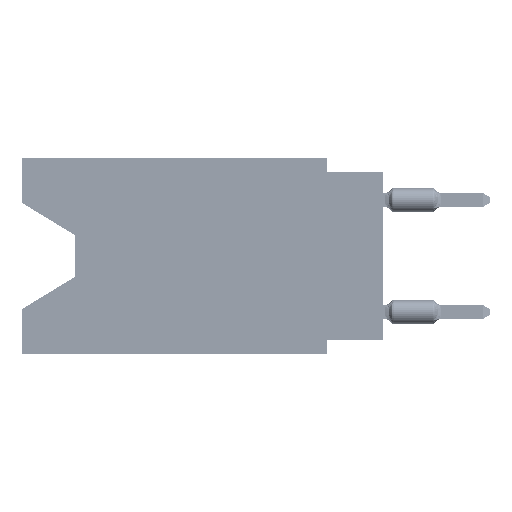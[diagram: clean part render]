
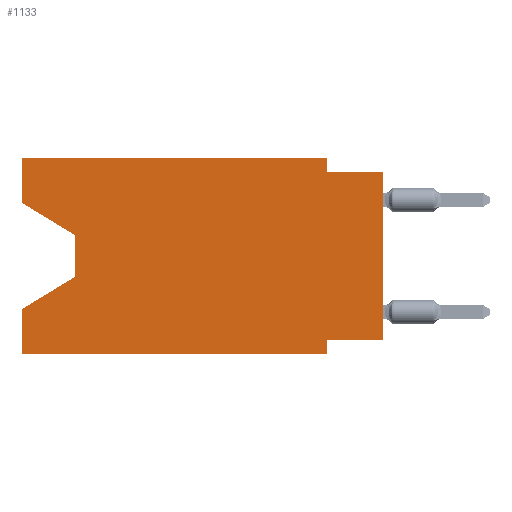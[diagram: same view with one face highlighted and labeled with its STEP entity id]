
A CAD part, left-side view. The second image highlights one B-rep face of the part: STEP entity #1133.
In plain terms, the highlighted planar face has unit normal (-1, 0, 0).
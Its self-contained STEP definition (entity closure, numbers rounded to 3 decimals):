
#1133 = ADVANCED_FACE ( 'NONE', ( #46735 ), #67381, .F. ) ;
#1563 = CARTESIAN_POINT ( 'NONE',  ( 0., 16.383, 0. ) ) ;
#1635 = CARTESIAN_POINT ( 'NONE',  ( 0., 0., -0.635 ) ) ;
#2254 = VERTEX_POINT ( 'NONE', #71745 ) ;
#2310 = VERTEX_POINT ( 'NONE', #57102 ) ;
#2483 = CARTESIAN_POINT ( 'NONE',  ( 0., 13.97, -5.385 ) ) ;
#3102 = VERTEX_POINT ( 'NONE', #33386 ) ;
#5741 = EDGE_LOOP ( 'NONE', ( #50713, #13413, #11217, #46353, #14247, #51278, #54764, #56738, #67167, #51960, #11838, #71206 ) ) ;
#6582 = EDGE_CURVE ( 'NONE', #58281, #15753, #70233, .T. ) ;
#9421 = VECTOR ( 'NONE', #40419, 1000. ) ;
#9939 = CARTESIAN_POINT ( 'NONE',  ( 0., 16.383, -6.852 ) ) ;
#10693 = LINE ( 'NONE', #43326, #68741 ) ;
#11217 = ORIENTED_EDGE ( 'NONE', *, *, #6582, .T. ) ;
#11391 = DIRECTION ( 'NONE',  ( 0., 0., -1. ) ) ;
#11838 = ORIENTED_EDGE ( 'NONE', *, *, #20810, .F. ) ;
#13413 = ORIENTED_EDGE ( 'NONE', *, *, #21229, .T. ) ;
#13521 = DIRECTION ( 'NONE',  ( 0., 0., 1. ) ) ;
#13876 = LINE ( 'NONE', #63709, #57979 ) ;
#14247 = ORIENTED_EDGE ( 'NONE', *, *, #32171, .T. ) ;
#14319 = CARTESIAN_POINT ( 'NONE',  ( 0., 16.383, -8.89 ) ) ;
#14470 = DIRECTION ( 'NONE',  ( 0., 0., -1. ) ) ;
#15527 = VECTOR ( 'NONE', #39495, 1000. ) ;
#15753 = VERTEX_POINT ( 'NONE', #9939 ) ;
#16280 = LINE ( 'NONE', #55493, #27519 ) ;
#16481 = VECTOR ( 'NONE', #11391, 1000. ) ;
#16884 = CARTESIAN_POINT ( 'NONE',  ( 0., 13.97, -3.505 ) ) ;
#20309 = CARTESIAN_POINT ( 'NONE',  ( 0., 13.97, -5.385 ) ) ;
#20413 = LINE ( 'NONE', #42416, #56230 ) ;
#20764 = EDGE_CURVE ( 'NONE', #67572, #26858, #44441, .T. ) ;
#20810 = EDGE_CURVE ( 'NONE', #54937, #67572, #62748, .T. ) ;
#21229 = EDGE_CURVE ( 'NONE', #2310, #58281, #67075, .T. ) ;
#21707 = DIRECTION ( 'NONE',  ( 0., 0., -1. ) ) ;
#22900 = DIRECTION ( 'NONE',  ( 0., -1., 0. ) ) ;
#23270 = EDGE_CURVE ( 'NONE', #3102, #2310, #48601, .T. ) ;
#24061 = VERTEX_POINT ( 'NONE', #40844 ) ;
#24678 = EDGE_CURVE ( 'NONE', #44753, #24061, #67694, .T. ) ;
#26858 = VERTEX_POINT ( 'NONE', #55972 ) ;
#27519 = VECTOR ( 'NONE', #22900, 1000. ) ;
#29062 = DIRECTION ( 'NONE',  ( 0., 0., -1. ) ) ;
#31744 = DIRECTION ( 'NONE',  ( 0., -0.855, -0.519 ) ) ;
#31796 = LINE ( 'NONE', #66209, #64848 ) ;
#32171 = EDGE_CURVE ( 'NONE', #32917, #2254, #16280, .T. ) ;
#32917 = VERTEX_POINT ( 'NONE', #14319 ) ;
#33373 = EDGE_CURVE ( 'NONE', #44753, #54329, #13876, .T. ) ;
#33386 = CARTESIAN_POINT ( 'NONE',  ( 0., 16.383, -2.038 ) ) ;
#35311 = EDGE_CURVE ( 'NONE', #24061, #2254, #10693, .T. ) ;
#36194 = DIRECTION ( 'NONE',  ( 0., -1., 0. ) ) ;
#39495 = DIRECTION ( 'NONE',  ( 0., 1., 0. ) ) ;
#39687 = CARTESIAN_POINT ( 'NONE',  ( 0., 2.54, 0. ) ) ;
#40357 = DIRECTION ( 'NONE',  ( 0., 0., 1. ) ) ;
#40419 = DIRECTION ( 'NONE',  ( 0., -1., 0. ) ) ;
#40844 = CARTESIAN_POINT ( 'NONE',  ( 0., 2.54, -8.255 ) ) ;
#42416 = CARTESIAN_POINT ( 'NONE',  ( 0., 0., -0.635 ) ) ;
#43326 = CARTESIAN_POINT ( 'NONE',  ( 0., 2.54, -8.89 ) ) ;
#43647 = CARTESIAN_POINT ( 'NONE',  ( 0., 16.383, 0. ) ) ;
#44067 = VECTOR ( 'NONE', #40357, 1000. ) ;
#44441 = LINE ( 'NONE', #61653, #64447 ) ;
#44753 = VERTEX_POINT ( 'NONE', #45412 ) ;
#44961 = EDGE_CURVE ( 'NONE', #32917, #15753, #31796, .T. ) ;
#45412 = CARTESIAN_POINT ( 'NONE',  ( 0., 0., -8.255 ) ) ;
#45782 = VECTOR ( 'NONE', #31744, 1000. ) ;
#46353 = ORIENTED_EDGE ( 'NONE', *, *, #44961, .F. ) ;
#46735 = FACE_OUTER_BOUND ( 'NONE', #5741, .T. ) ;
#48601 = LINE ( 'NONE', #54821, #45782 ) ;
#48630 = DIRECTION ( 'NONE',  ( 0., 0.855, -0.519 ) ) ;
#48861 = EDGE_CURVE ( 'NONE', #3102, #54937, #68188, .T. ) ;
#50713 = ORIENTED_EDGE ( 'NONE', *, *, #23270, .T. ) ;
#51278 = ORIENTED_EDGE ( 'NONE', *, *, #35311, .F. ) ;
#51960 = ORIENTED_EDGE ( 'NONE', *, *, #20764, .F. ) ;
#54329 = VERTEX_POINT ( 'NONE', #1635 ) ;
#54764 = ORIENTED_EDGE ( 'NONE', *, *, #24678, .F. ) ;
#54765 = DIRECTION ( 'NONE',  ( 1., 0., 0. ) ) ;
#54821 = CARTESIAN_POINT ( 'NONE',  ( 0., 16.383, -2.038 ) ) ;
#54937 = VERTEX_POINT ( 'NONE', #43647 ) ;
#55493 = CARTESIAN_POINT ( 'NONE',  ( 0., 16.383, -8.89 ) ) ;
#55972 = CARTESIAN_POINT ( 'NONE',  ( 0., 2.54, -0.635 ) ) ;
#56124 = AXIS2_PLACEMENT_3D ( 'NONE', #69084, #54765, #14470 ) ;
#56230 = VECTOR ( 'NONE', #36194, 1000. ) ;
#56703 = CARTESIAN_POINT ( 'NONE',  ( 0., 0., -8.255 ) ) ;
#56738 = ORIENTED_EDGE ( 'NONE', *, *, #33373, .T. ) ;
#57102 = CARTESIAN_POINT ( 'NONE',  ( 0., 13.97, -3.505 ) ) ;
#57979 = VECTOR ( 'NONE', #13521, 1000. ) ;
#58281 = VERTEX_POINT ( 'NONE', #20309 ) ;
#61297 = VECTOR ( 'NONE', #48630, 1000. ) ;
#61653 = CARTESIAN_POINT ( 'NONE',  ( 0., 2.54, 0. ) ) ;
#62748 = LINE ( 'NONE', #1563, #9421 ) ;
#63709 = CARTESIAN_POINT ( 'NONE',  ( 0., 0., 0. ) ) ;
#64435 = EDGE_CURVE ( 'NONE', #26858, #54329, #20413, .T. ) ;
#64447 = VECTOR ( 'NONE', #29062, 1000. ) ;
#64766 = DIRECTION ( 'NONE',  ( 0., 0., 1. ) ) ;
#64848 = VECTOR ( 'NONE', #64766, 1000. ) ;
#66209 = CARTESIAN_POINT ( 'NONE',  ( 0., 16.383, 0. ) ) ;
#67075 = LINE ( 'NONE', #16884, #16481 ) ;
#67167 = ORIENTED_EDGE ( 'NONE', *, *, #64435, .F. ) ;
#67381 = PLANE ( 'NONE',  #56124 ) ;
#67572 = VERTEX_POINT ( 'NONE', #39687 ) ;
#67694 = LINE ( 'NONE', #56703, #15527 ) ;
#67827 = CARTESIAN_POINT ( 'NONE',  ( 0., 16.383, 0. ) ) ;
#68188 = LINE ( 'NONE', #67827, #44067 ) ;
#68741 = VECTOR ( 'NONE', #21707, 1000. ) ;
#69084 = CARTESIAN_POINT ( 'NONE',  ( 0., 16.383, 0. ) ) ;
#70233 = LINE ( 'NONE', #2483, #61297 ) ;
#71206 = ORIENTED_EDGE ( 'NONE', *, *, #48861, .F. ) ;
#71745 = CARTESIAN_POINT ( 'NONE',  ( 0., 2.54, -8.89 ) ) ;
